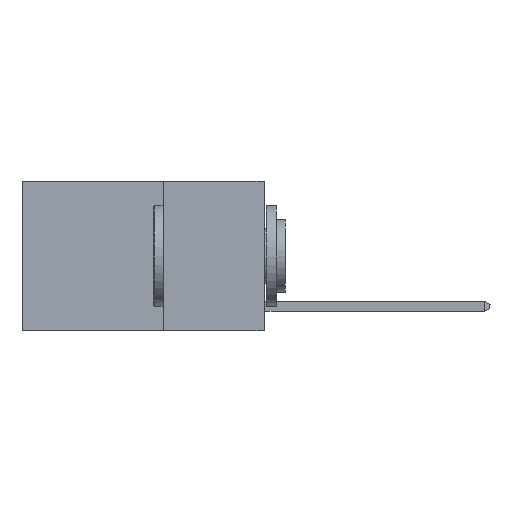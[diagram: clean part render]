
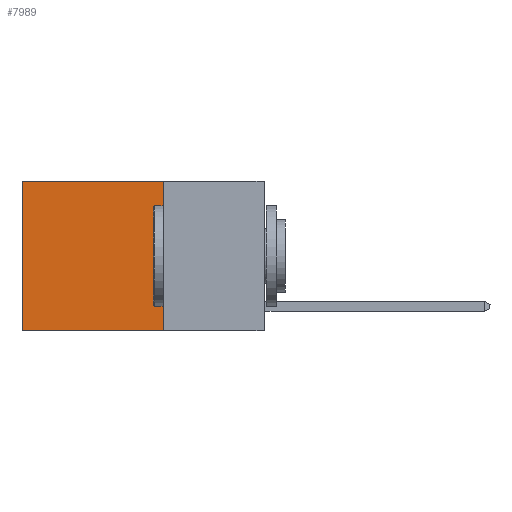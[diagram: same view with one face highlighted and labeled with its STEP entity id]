
A CAD part, left-side view. The second image highlights one B-rep face of the part: STEP entity #7989.
In plain terms, the highlighted planar face has unit normal (-1, 0, 0).
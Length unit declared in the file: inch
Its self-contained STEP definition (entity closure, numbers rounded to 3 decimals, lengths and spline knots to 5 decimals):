
#212 = VECTOR ( 'NONE', #1889, 39.37008 ) ;
#1679 = EDGE_CURVE ( 'NONE', #13810, #13609, #13805, .T. ) ;
#1889 = DIRECTION ( 'NONE',  ( 0., 0., -1. ) ) ;
#2632 = ORIENTED_EDGE ( 'NONE', *, *, #9793, .F. ) ;
#3117 = CARTESIAN_POINT ( 'NONE',  ( 0.2625, 0.6, -0.37 ) ) ;
#3312 = AXIS2_PLACEMENT_3D ( 'NONE', #16971, #5925, #15651 ) ;
#3885 = LINE ( 'NONE', #15768, #212 ) ;
#5452 = EDGE_LOOP ( 'NONE', ( #5893, #13313, #2632, #6343 ) ) ;
#5711 = VECTOR ( 'NONE', #9639, 39.37008 ) ;
#5893 = ORIENTED_EDGE ( 'NONE', *, *, #7205, .T. ) ;
#5925 = DIRECTION ( 'NONE',  ( 1., 0., 0. ) ) ;
#6343 = ORIENTED_EDGE ( 'NONE', *, *, #8345, .T. ) ;
#6405 = VECTOR ( 'NONE', #10906, 39.37008 ) ;
#6693 = DIRECTION ( 'NONE',  ( 0., 0., -1. ) ) ;
#7205 = EDGE_CURVE ( 'NONE', #17418, #13609, #16378, .T. ) ;
#7251 = FACE_OUTER_BOUND ( 'NONE', #5452, .T. ) ;
#7989 = ADVANCED_FACE ( 'NONE', ( #7251 ), #11456, .F. ) ;
#8329 = VERTEX_POINT ( 'NONE', #13775 ) ;
#8336 = CARTESIAN_POINT ( 'NONE',  ( 0.2625, 0.6, 0. ) ) ;
#8345 = EDGE_CURVE ( 'NONE', #8329, #17418, #17200, .T. ) ;
#8964 = VECTOR ( 'NONE', #6693, 39.37008 ) ;
#9639 = DIRECTION ( 'NONE',  ( 0., 1., 0. ) ) ;
#9793 = EDGE_CURVE ( 'NONE', #8329, #13810, #3885, .T. ) ;
#10906 = DIRECTION ( 'NONE',  ( 0., 1., 0. ) ) ;
#11456 = PLANE ( 'NONE',  #3312 ) ;
#11941 = CARTESIAN_POINT ( 'NONE',  ( 0.2625, 0.25, -0.37 ) ) ;
#13313 = ORIENTED_EDGE ( 'NONE', *, *, #1679, .F. ) ;
#13609 = VERTEX_POINT ( 'NONE', #3117 ) ;
#13775 = CARTESIAN_POINT ( 'NONE',  ( 0.2625, 0.25, 0. ) ) ;
#13805 = LINE ( 'NONE', #17787, #6405 ) ;
#13810 = VERTEX_POINT ( 'NONE', #11941 ) ;
#15019 = CARTESIAN_POINT ( 'NONE',  ( 0.2625, 0.6, 0. ) ) ;
#15234 = CARTESIAN_POINT ( 'NONE',  ( 0.2625, 0.25, 0. ) ) ;
#15651 = DIRECTION ( 'NONE',  ( 0., 0., -1. ) ) ;
#15768 = CARTESIAN_POINT ( 'NONE',  ( 0.2625, 0.25, 0. ) ) ;
#16378 = LINE ( 'NONE', #15019, #8964 ) ;
#16971 = CARTESIAN_POINT ( 'NONE',  ( 0.2625, 0.25, 0. ) ) ;
#17200 = LINE ( 'NONE', #15234, #5711 ) ;
#17418 = VERTEX_POINT ( 'NONE', #8336 ) ;
#17787 = CARTESIAN_POINT ( 'NONE',  ( 0.2625, 0.25, -0.37 ) ) ;
